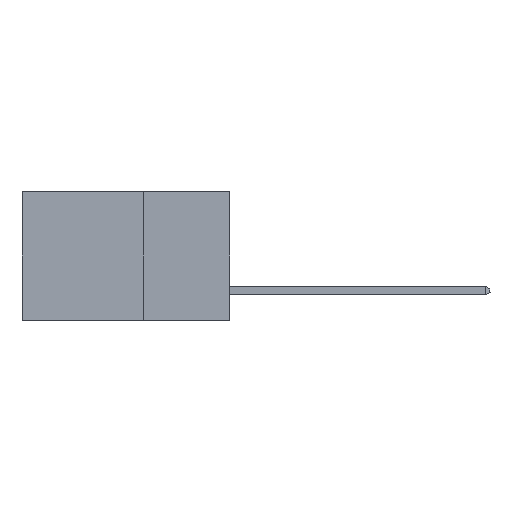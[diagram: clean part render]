
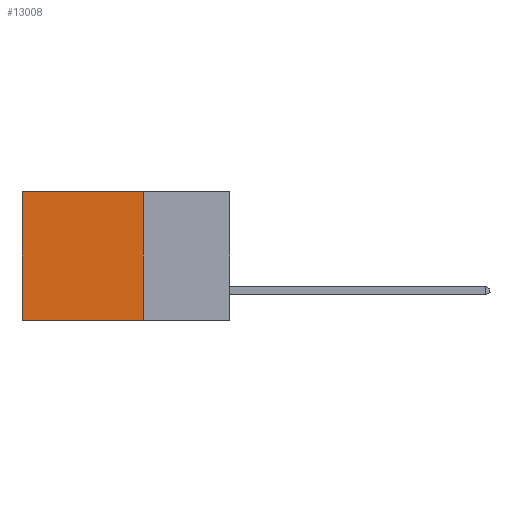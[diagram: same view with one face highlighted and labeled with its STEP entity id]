
A CAD part, left-side view. The second image highlights one B-rep face of the part: STEP entity #13008.
In plain terms, the highlighted planar face has unit normal (-1, 0, 0).
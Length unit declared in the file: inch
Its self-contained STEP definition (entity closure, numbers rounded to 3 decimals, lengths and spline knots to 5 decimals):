
#780 = ORIENTED_EDGE ( 'NONE', *, *, #11327, .T. ) ;
#1984 = CARTESIAN_POINT ( 'NONE',  ( 0.298, 0.6, 0. ) ) ;
#2489 = CARTESIAN_POINT ( 'NONE',  ( 0.298, 0.6, 0. ) ) ;
#2851 = EDGE_LOOP ( 'NONE', ( #780, #8928, #7828, #9620 ) ) ;
#2904 = VECTOR ( 'NONE', #12974, 39.37008 ) ;
#2990 = VECTOR ( 'NONE', #4438, 39.37008 ) ;
#4438 = DIRECTION ( 'NONE',  ( 0., 0., -1. ) ) ;
#5370 = CARTESIAN_POINT ( 'NONE',  ( 0.298, 0.25, -0.37 ) ) ;
#5466 = EDGE_CURVE ( 'NONE', #16829, #19151, #15762, .T. ) ;
#7292 = VERTEX_POINT ( 'NONE', #11088 ) ;
#7828 = ORIENTED_EDGE ( 'NONE', *, *, #5466, .F. ) ;
#8928 = ORIENTED_EDGE ( 'NONE', *, *, #12254, .F. ) ;
#9267 = FACE_OUTER_BOUND ( 'NONE', #2851, .T. ) ;
#9580 = VECTOR ( 'NONE', #12654, 39.37008 ) ;
#9620 = ORIENTED_EDGE ( 'NONE', *, *, #12201, .T. ) ;
#10416 = DIRECTION ( 'NONE',  ( 1., 0., 0. ) ) ;
#10971 = CARTESIAN_POINT ( 'NONE',  ( 0.298, 0.25, 0. ) ) ;
#11088 = CARTESIAN_POINT ( 'NONE',  ( 0.298, 0.6, -0.37 ) ) ;
#11327 = EDGE_CURVE ( 'NONE', #18771, #7292, #18097, .T. ) ;
#11736 = AXIS2_PLACEMENT_3D ( 'NONE', #19335, #10416, #14842 ) ;
#12201 = EDGE_CURVE ( 'NONE', #16829, #18771, #12827, .T. ) ;
#12254 = EDGE_CURVE ( 'NONE', #19151, #7292, #19444, .T. ) ;
#12317 = CARTESIAN_POINT ( 'NONE',  ( 0.298, 0.25, -0.37 ) ) ;
#12595 = VECTOR ( 'NONE', #17548, 39.37008 ) ;
#12654 = DIRECTION ( 'NONE',  ( 0., 0., -1. ) ) ;
#12827 = LINE ( 'NONE', #16025, #2904 ) ;
#12974 = DIRECTION ( 'NONE',  ( 0., 1., 0. ) ) ;
#13008 = ADVANCED_FACE ( 'NONE', ( #9267 ), #14917, .F. ) ;
#14842 = DIRECTION ( 'NONE',  ( 0., 0., -1. ) ) ;
#14917 = PLANE ( 'NONE',  #11736 ) ;
#15762 = LINE ( 'NONE', #17933, #2990 ) ;
#16025 = CARTESIAN_POINT ( 'NONE',  ( 0.298, 0.25, 0. ) ) ;
#16829 = VERTEX_POINT ( 'NONE', #10971 ) ;
#17548 = DIRECTION ( 'NONE',  ( 0., 1., 0. ) ) ;
#17933 = CARTESIAN_POINT ( 'NONE',  ( 0.298, 0.25, 0. ) ) ;
#18097 = LINE ( 'NONE', #1984, #9580 ) ;
#18771 = VERTEX_POINT ( 'NONE', #2489 ) ;
#19151 = VERTEX_POINT ( 'NONE', #12317 ) ;
#19335 = CARTESIAN_POINT ( 'NONE',  ( 0.298, 0.25, 0. ) ) ;
#19444 = LINE ( 'NONE', #5370, #12595 ) ;
